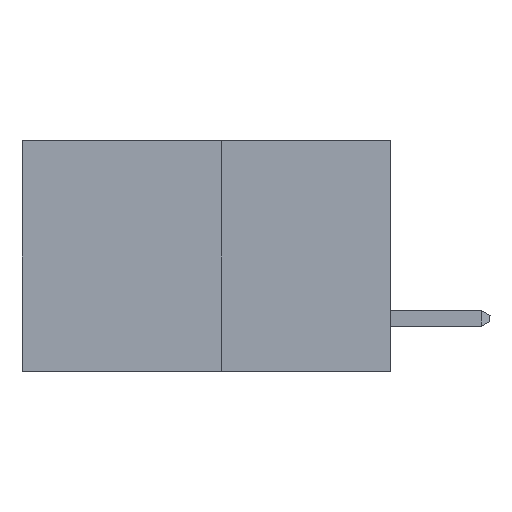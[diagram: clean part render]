
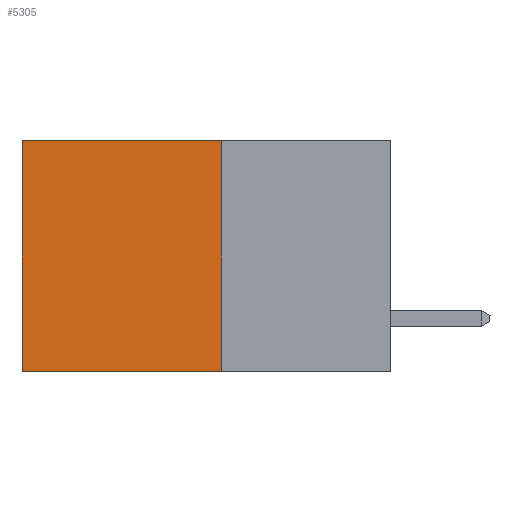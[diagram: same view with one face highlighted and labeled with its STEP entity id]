
A CAD part, left-side view. The second image highlights one B-rep face of the part: STEP entity #5305.
In plain terms, the highlighted planar face has unit normal (-1, 0, 0).
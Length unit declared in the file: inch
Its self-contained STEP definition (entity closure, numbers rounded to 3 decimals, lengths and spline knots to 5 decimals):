
#1819 = VECTOR ( 'NONE', #5667, 39.37008 ) ;
#2442 = ORIENTED_EDGE ( 'NONE', *, *, #10886, .T. ) ;
#2850 = ORIENTED_EDGE ( 'NONE', *, *, #16222, .F. ) ;
#3269 = EDGE_LOOP ( 'NONE', ( #2442, #2850, #3817, #4219 ) ) ;
#3817 = ORIENTED_EDGE ( 'NONE', *, *, #5341, .F. ) ;
#4168 = CARTESIAN_POINT ( 'NONE',  ( 0.277, 0.27, -0.37 ) ) ;
#4219 = ORIENTED_EDGE ( 'NONE', *, *, #12822, .T. ) ;
#4296 = CARTESIAN_POINT ( 'NONE',  ( 0.277, 0.27, 0. ) ) ;
#4360 = CARTESIAN_POINT ( 'NONE',  ( 0.277, 0.59, 0. ) ) ;
#4499 = LINE ( 'NONE', #10068, #11256 ) ;
#4855 = AXIS2_PLACEMENT_3D ( 'NONE', #10662, #10543, #10495 ) ;
#4934 = FACE_OUTER_BOUND ( 'NONE', #3269, .T. ) ;
#5247 = VERTEX_POINT ( 'NONE', #11540 ) ;
#5305 = ADVANCED_FACE ( 'NONE', ( #4934 ), #10919, .F. ) ;
#5341 = EDGE_CURVE ( 'NONE', #5247, #9753, #4499, .T. ) ;
#5667 = DIRECTION ( 'NONE',  ( 0., 1., 0. ) ) ;
#8070 = CARTESIAN_POINT ( 'NONE',  ( 0.277, 0.59, -0.37 ) ) ;
#8855 = CARTESIAN_POINT ( 'NONE',  ( 0.277, 0.59, -0.37 ) ) ;
#9425 = VECTOR ( 'NONE', #16122, 39.37008 ) ;
#9594 = CARTESIAN_POINT ( 'NONE',  ( 0.277, 0.27, -0.37 ) ) ;
#9753 = VERTEX_POINT ( 'NONE', #4168 ) ;
#9787 = DIRECTION ( 'NONE',  ( 0., 0., -1. ) ) ;
#9863 = LINE ( 'NONE', #9594, #9425 ) ;
#10068 = CARTESIAN_POINT ( 'NONE',  ( 0.277, 0.27, -0.37 ) ) ;
#10495 = DIRECTION ( 'NONE',  ( 0., 0., -1. ) ) ;
#10543 = DIRECTION ( 'NONE',  ( 1., 0., 0. ) ) ;
#10662 = CARTESIAN_POINT ( 'NONE',  ( 0.277, 0.27, -0.37 ) ) ;
#10886 = EDGE_CURVE ( 'NONE', #16313, #15844, #17184, .T. ) ;
#10919 = PLANE ( 'NONE',  #4855 ) ;
#11256 = VECTOR ( 'NONE', #9787, 39.37008 ) ;
#11540 = CARTESIAN_POINT ( 'NONE',  ( 0.277, 0.27, 0. ) ) ;
#12822 = EDGE_CURVE ( 'NONE', #5247, #16313, #13067, .T. ) ;
#13067 = LINE ( 'NONE', #4296, #1819 ) ;
#15844 = VERTEX_POINT ( 'NONE', #8855 ) ;
#15975 = DIRECTION ( 'NONE',  ( 0., 0., -1. ) ) ;
#16122 = DIRECTION ( 'NONE',  ( 0., 1., 0. ) ) ;
#16222 = EDGE_CURVE ( 'NONE', #9753, #15844, #9863, .T. ) ;
#16313 = VERTEX_POINT ( 'NONE', #4360 ) ;
#16387 = VECTOR ( 'NONE', #15975, 39.37008 ) ;
#17184 = LINE ( 'NONE', #8070, #16387 ) ;
